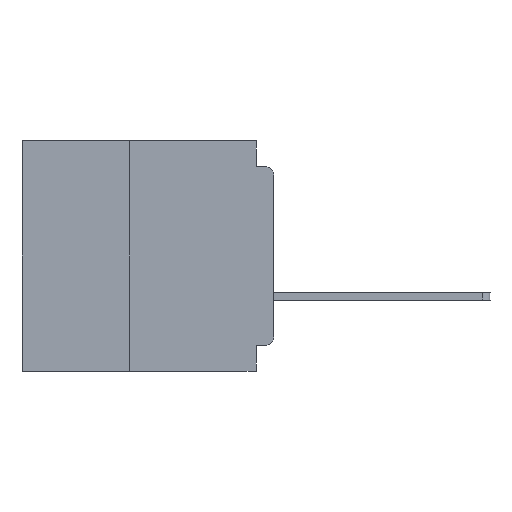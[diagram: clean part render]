
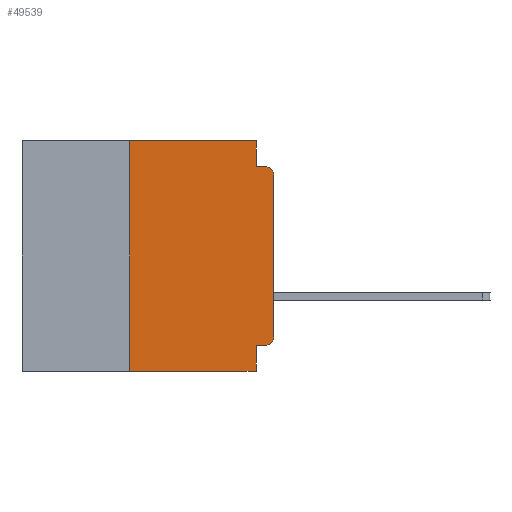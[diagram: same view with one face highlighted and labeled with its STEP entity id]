
A CAD part, left-side view. The second image highlights one B-rep face of the part: STEP entity #49539.
In plain terms, the highlighted planar face has unit normal (-1, 0, 0).
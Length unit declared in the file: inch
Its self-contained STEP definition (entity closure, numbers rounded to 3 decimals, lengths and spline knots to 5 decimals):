
#940 = CARTESIAN_POINT ( 'NONE',  ( 0., 0.015, -0.045 ) ) ;
#1902 = CIRCLE ( 'NONE', #29985, 0.015 ) ;
#2440 = EDGE_CURVE ( 'NONE', #32542, #6286, #48885, .T. ) ;
#2659 = CARTESIAN_POINT ( 'NONE',  ( 0., 0.031, -0.045 ) ) ;
#3314 = VECTOR ( 'NONE', #45743, 39.37008 ) ;
#3637 = EDGE_CURVE ( 'NONE', #31011, #6286, #9429, .T. ) ;
#4183 = VERTEX_POINT ( 'NONE', #5590 ) ;
#5590 = CARTESIAN_POINT ( 'NONE',  ( 0., 0.031, -0.4 ) ) ;
#5797 = VERTEX_POINT ( 'NONE', #14780 ) ;
#6199 = DIRECTION ( 'NONE',  ( 0., 0., 1. ) ) ;
#6286 = VERTEX_POINT ( 'NONE', #940 ) ;
#7629 = EDGE_CURVE ( 'NONE', #50693, #45030, #1902, .T. ) ;
#8669 = LINE ( 'NONE', #37625, #54977 ) ;
#9273 = LINE ( 'NONE', #44586, #55553 ) ;
#9429 = LINE ( 'NONE', #46282, #33354 ) ;
#10485 = LINE ( 'NONE', #46455, #34371 ) ;
#11221 = LINE ( 'NONE', #44095, #30932 ) ;
#11433 = DIRECTION ( 'NONE',  ( 0., 0., -1. ) ) ;
#14448 = CARTESIAN_POINT ( 'NONE',  ( 0., 0.015, -0.34 ) ) ;
#14701 = ORIENTED_EDGE ( 'NONE', *, *, #57801, .F. ) ;
#14764 = EDGE_CURVE ( 'NONE', #5797, #31011, #16014, .T. ) ;
#14780 = CARTESIAN_POINT ( 'NONE',  ( 0., 0.031, 0. ) ) ;
#16014 = LINE ( 'NONE', #33818, #38424 ) ;
#16119 = FACE_OUTER_BOUND ( 'NONE', #46249, .T. ) ;
#16512 = CARTESIAN_POINT ( 'NONE',  ( 0., 0., -0.34 ) ) ;
#17576 = LINE ( 'NONE', #52265, #28177 ) ;
#17781 = DIRECTION ( 'NONE',  ( 0., -1., 0. ) ) ;
#18971 = DIRECTION ( 'NONE',  ( 0., 0., -1. ) ) ;
#19003 = CARTESIAN_POINT ( 'NONE',  ( 0., 0.25, 0. ) ) ;
#19633 = DIRECTION ( 'NONE',  ( 0., 0., -1. ) ) ;
#24099 = CARTESIAN_POINT ( 'NONE',  ( 0., 0.031, -0.355 ) ) ;
#24327 = DIRECTION ( 'NONE',  ( 0., 0., -1. ) ) ;
#24632 = ORIENTED_EDGE ( 'NONE', *, *, #43905, .F. ) ;
#26182 = EDGE_CURVE ( 'NONE', #46716, #4183, #11221, .T. ) ;
#27997 = CARTESIAN_POINT ( 'NONE',  ( 0., 0.25, -0.4 ) ) ;
#28177 = VECTOR ( 'NONE', #30000, 39.37008 ) ;
#28649 = CARTESIAN_POINT ( 'NONE',  ( 0., 0.437, 0. ) ) ;
#29985 = AXIS2_PLACEMENT_3D ( 'NONE', #14448, #45781, #18971 ) ;
#30000 = DIRECTION ( 'NONE',  ( 0., 1., 0. ) ) ;
#30011 = ORIENTED_EDGE ( 'NONE', *, *, #37386, .T. ) ;
#30932 = VECTOR ( 'NONE', #57571, 39.37008 ) ;
#31011 = VERTEX_POINT ( 'NONE', #2659 ) ;
#32483 = AXIS2_PLACEMENT_3D ( 'NONE', #28649, #51089, #24327 ) ;
#32542 = VERTEX_POINT ( 'NONE', #35209 ) ;
#32605 = CARTESIAN_POINT ( 'NONE',  ( 0., 0.015, -0.355 ) ) ;
#33354 = VECTOR ( 'NONE', #46156, 39.37008 ) ;
#33818 = CARTESIAN_POINT ( 'NONE',  ( 0., 0.031, 0. ) ) ;
#34371 = VECTOR ( 'NONE', #19633, 39.37008 ) ;
#34601 = VERTEX_POINT ( 'NONE', #24099 ) ;
#35209 = CARTESIAN_POINT ( 'NONE',  ( 0., 0., -0.06 ) ) ;
#36791 = ORIENTED_EDGE ( 'NONE', *, *, #26182, .T. ) ;
#37386 = EDGE_CURVE ( 'NONE', #45030, #32542, #8669, .T. ) ;
#37625 = CARTESIAN_POINT ( 'NONE',  ( 0., 0., 0. ) ) ;
#38424 = VECTOR ( 'NONE', #11433, 39.37008 ) ;
#38431 = CARTESIAN_POINT ( 'NONE',  ( 0., 0.25, -0.4 ) ) ;
#39077 = EDGE_CURVE ( 'NONE', #57182, #5797, #9273, .T. ) ;
#39733 = ORIENTED_EDGE ( 'NONE', *, *, #2440, .T. ) ;
#40760 = ORIENTED_EDGE ( 'NONE', *, *, #39077, .F. ) ;
#40974 = AXIS2_PLACEMENT_3D ( 'NONE', #47427, #47393, #47320 ) ;
#43905 = EDGE_CURVE ( 'NONE', #50693, #34601, #17576, .T. ) ;
#44095 = CARTESIAN_POINT ( 'NONE',  ( 0., 0.437, -0.4 ) ) ;
#44586 = CARTESIAN_POINT ( 'NONE',  ( 0., 0.437, 0. ) ) ;
#45030 = VERTEX_POINT ( 'NONE', #16512 ) ;
#45743 = DIRECTION ( 'NONE',  ( 0., 0., 1. ) ) ;
#45781 = DIRECTION ( 'NONE',  ( -1., 0., 0. ) ) ;
#46156 = DIRECTION ( 'NONE',  ( 0., -1., 0. ) ) ;
#46249 = EDGE_LOOP ( 'NONE', ( #30011, #39733, #58221, #50402, #40760, #14701, #36791, #57403, #24632, #57818 ) ) ;
#46282 = CARTESIAN_POINT ( 'NONE',  ( 0., 0., -0.045 ) ) ;
#46455 = CARTESIAN_POINT ( 'NONE',  ( 0., 0.031, -0.4 ) ) ;
#46573 = PLANE ( 'NONE',  #32483 ) ;
#46716 = VERTEX_POINT ( 'NONE', #38431 ) ;
#47320 = DIRECTION ( 'NONE',  ( 0., 0., -1. ) ) ;
#47393 = DIRECTION ( 'NONE',  ( -1., 0., 0. ) ) ;
#47427 = CARTESIAN_POINT ( 'NONE',  ( 0., 0.015, -0.06 ) ) ;
#48885 = CIRCLE ( 'NONE', #40974, 0.015 ) ;
#49539 = ADVANCED_FACE ( 'NONE', ( #16119 ), #46573, .F. ) ;
#50402 = ORIENTED_EDGE ( 'NONE', *, *, #14764, .F. ) ;
#50693 = VERTEX_POINT ( 'NONE', #32605 ) ;
#51089 = DIRECTION ( 'NONE',  ( 1., 0., 0. ) ) ;
#51126 = LINE ( 'NONE', #27997, #3314 ) ;
#52265 = CARTESIAN_POINT ( 'NONE',  ( 0., 0., -0.355 ) ) ;
#54977 = VECTOR ( 'NONE', #6199, 39.37008 ) ;
#55553 = VECTOR ( 'NONE', #17781, 39.37008 ) ;
#56624 = EDGE_CURVE ( 'NONE', #34601, #4183, #10485, .T. ) ;
#57182 = VERTEX_POINT ( 'NONE', #19003 ) ;
#57403 = ORIENTED_EDGE ( 'NONE', *, *, #56624, .F. ) ;
#57571 = DIRECTION ( 'NONE',  ( 0., -1., 0. ) ) ;
#57801 = EDGE_CURVE ( 'NONE', #46716, #57182, #51126, .T. ) ;
#57818 = ORIENTED_EDGE ( 'NONE', *, *, #7629, .T. ) ;
#58221 = ORIENTED_EDGE ( 'NONE', *, *, #3637, .F. ) ;
